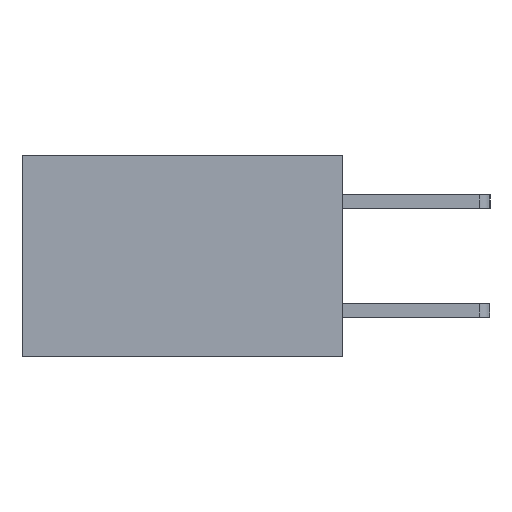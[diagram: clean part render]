
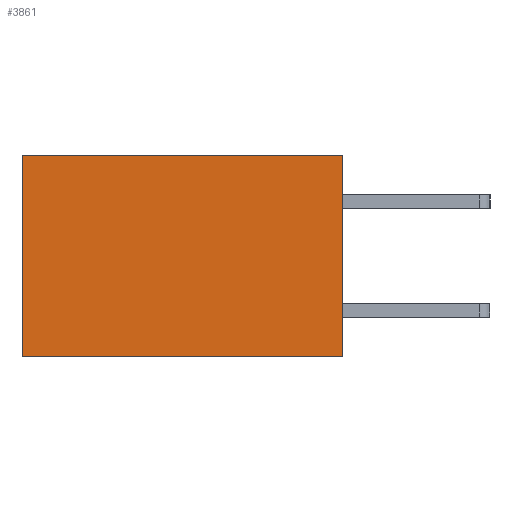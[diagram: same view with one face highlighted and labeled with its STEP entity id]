
A CAD part, left-side view. The second image highlights one B-rep face of the part: STEP entity #3861.
In plain terms, the highlighted planar face has unit normal (-1, 0, 0).
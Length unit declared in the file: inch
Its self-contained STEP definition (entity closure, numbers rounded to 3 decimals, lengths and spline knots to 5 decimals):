
#732 = EDGE_CURVE ( 'NONE', #4707, #5166, #9802, .T. ) ;
#1083 = ORIENTED_EDGE ( 'NONE', *, *, #3978, .T. ) ;
#1446 = DIRECTION ( 'NONE',  ( 0., 1., 0. ) ) ;
#2104 = CARTESIAN_POINT ( 'NONE',  ( 0.277, 0., -0.37 ) ) ;
#2137 = VECTOR ( 'NONE', #1446, 39.37008 ) ;
#2252 = DIRECTION ( 'NONE',  ( 1., 0., 0. ) ) ;
#2594 = ORIENTED_EDGE ( 'NONE', *, *, #3697, .F. ) ;
#3228 = CARTESIAN_POINT ( 'NONE',  ( 0.277, 0.59, -0.37 ) ) ;
#3697 = EDGE_CURVE ( 'NONE', #5440, #10222, #5336, .T. ) ;
#3840 = ORIENTED_EDGE ( 'NONE', *, *, #732, .T. ) ;
#3861 = ADVANCED_FACE ( 'NONE', ( #7408 ), #6402, .F. ) ;
#3978 = EDGE_CURVE ( 'NONE', #5440, #4707, #5019, .T. ) ;
#4707 = VERTEX_POINT ( 'NONE', #7931 ) ;
#4912 = LINE ( 'NONE', #2104, #7162 ) ;
#5019 = LINE ( 'NONE', #8517, #2137 ) ;
#5031 = VECTOR ( 'NONE', #12462, 39.37008 ) ;
#5166 = VERTEX_POINT ( 'NONE', #7651 ) ;
#5336 = LINE ( 'NONE', #5949, #5031 ) ;
#5440 = VERTEX_POINT ( 'NONE', #8803 ) ;
#5685 = EDGE_CURVE ( 'NONE', #10222, #5166, #4912, .T. ) ;
#5949 = CARTESIAN_POINT ( 'NONE',  ( 0.277, 0., -0.37 ) ) ;
#6402 = PLANE ( 'NONE',  #10678 ) ;
#7162 = VECTOR ( 'NONE', #9054, 39.37008 ) ;
#7297 = CARTESIAN_POINT ( 'NONE',  ( 0.277, 0., -0.37 ) ) ;
#7343 = VECTOR ( 'NONE', #10639, 39.37008 ) ;
#7408 = FACE_OUTER_BOUND ( 'NONE', #10250, .T. ) ;
#7651 = CARTESIAN_POINT ( 'NONE',  ( 0.277, 0.59, -0.37 ) ) ;
#7931 = CARTESIAN_POINT ( 'NONE',  ( 0.277, 0.59, 0. ) ) ;
#8233 = CARTESIAN_POINT ( 'NONE',  ( 0.277, 0., -0.37 ) ) ;
#8517 = CARTESIAN_POINT ( 'NONE',  ( 0.277, 0., 0. ) ) ;
#8803 = CARTESIAN_POINT ( 'NONE',  ( 0.277, 0., 0. ) ) ;
#9054 = DIRECTION ( 'NONE',  ( 0., 1., 0. ) ) ;
#9182 = DIRECTION ( 'NONE',  ( 0., 0., -1. ) ) ;
#9802 = LINE ( 'NONE', #3228, #7343 ) ;
#10222 = VERTEX_POINT ( 'NONE', #7297 ) ;
#10250 = EDGE_LOOP ( 'NONE', ( #3840, #12028, #2594, #1083 ) ) ;
#10639 = DIRECTION ( 'NONE',  ( 0., 0., -1. ) ) ;
#10678 = AXIS2_PLACEMENT_3D ( 'NONE', #8233, #2252, #9182 ) ;
#12028 = ORIENTED_EDGE ( 'NONE', *, *, #5685, .F. ) ;
#12462 = DIRECTION ( 'NONE',  ( 0., 0., -1. ) ) ;
